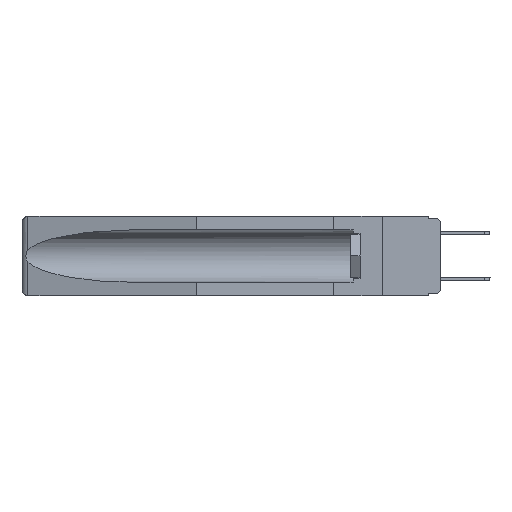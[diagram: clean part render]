
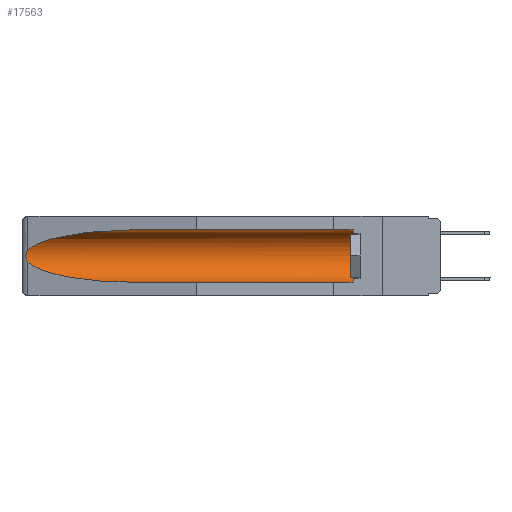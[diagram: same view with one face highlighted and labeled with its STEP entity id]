
A CAD part, left-side view. The second image highlights one B-rep face of the part: STEP entity #17563.
In plain terms, the highlighted cylindrical face has radius 2.857 mm (diameter 5.715 mm), a partial arc.
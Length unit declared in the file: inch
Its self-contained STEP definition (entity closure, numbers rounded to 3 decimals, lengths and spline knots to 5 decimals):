
#345 = EDGE_CURVE ( 'NONE', #7785, #2218, #491, .T. ) ;
#491 =( BOUNDED_CURVE ( )  B_SPLINE_CURVE ( 3, ( #11418, #5272, #18903, #6684 ),
 .UNSPECIFIED., .F., .F. ) 
 B_SPLINE_CURVE_WITH_KNOTS ( ( 4, 4 ),
 ( 4.71239, 6.08839 ),
 .UNSPECIFIED. ) 
 CURVE ( )  GEOMETRIC_REPRESENTATION_ITEM ( )  RATIONAL_B_SPLINE_CURVE ( ( 1., 0.848, 0.848, 1. ) ) 
 REPRESENTATION_ITEM ( '' )  );
#539 = VECTOR ( 'NONE', #11460, 39.37008 ) ;
#713 = CARTESIAN_POINT ( 'NONE',  ( 0.155, -0.30754, -0.284 ) ) ;
#914 = EDGE_CURVE ( 'NONE', #5706, #6888, #1762, .T. ) ;
#940 = EDGE_CURVE ( 'NONE', #5706, #18076, #4893, .T. ) ;
#1762 = CIRCLE ( 'NONE', #2963, 0.1125 ) ;
#1925 = LINE ( 'NONE', #9949, #17726 ) ;
#2218 = VERTEX_POINT ( 'NONE', #7419 ) ;
#2226 = DIRECTION ( 'NONE',  ( 0., 0., 1. ) ) ;
#2325 = DIRECTION ( 'NONE',  ( 0., 0., 1. ) ) ;
#2847 = CARTESIAN_POINT ( 'NONE',  ( 0.26537, 1.52718, -0.19328 ) ) ;
#2963 = AXIS2_PLACEMENT_3D ( 'NONE', #9897, #11526, #2226 ) ;
#3067 = CARTESIAN_POINT ( 'NONE',  ( 0.26537, 1.52718, -0.19328 ) ) ;
#3264 = EDGE_CURVE ( 'NONE', #6962, #18076, #4589, .T. ) ;
#3426 = AXIS2_PLACEMENT_3D ( 'NONE', #16192, #5473, #2325 ) ;
#4138 = EDGE_CURVE ( 'NONE', #2218, #6962, #8749, .T. ) ;
#4213 = CARTESIAN_POINT ( 'NONE',  ( 0.155, 0.126, -0.059 ) ) ;
#4589 =( BOUNDED_CURVE ( )  B_SPLINE_CURVE ( 3, ( #16500, #5777, #8777, #11725 ),
 .UNSPECIFIED., .F., .F. ) 
 B_SPLINE_CURVE_WITH_KNOTS ( ( 4, 4 ),
 ( 0.1948, 1.5708 ),
 .UNSPECIFIED. ) 
 CURVE ( )  GEOMETRIC_REPRESENTATION_ITEM ( )  RATIONAL_B_SPLINE_CURVE ( ( 1., 0.848, 0.848, 1. ) ) 
 REPRESENTATION_ITEM ( '' )  );
#4893 = LINE ( 'NONE', #713, #539 ) ;
#4951 = ORIENTED_EDGE ( 'NONE', *, *, #345, .T. ) ;
#4993 = ORIENTED_EDGE ( 'NONE', *, *, #940, .F. ) ;
#5272 = CARTESIAN_POINT ( 'NONE',  ( 0.21114, 1.30732, -0.059 ) ) ;
#5427 = DIRECTION ( 'NONE',  ( 0., 1., 0. ) ) ;
#5473 = DIRECTION ( 'NONE',  ( 0., 1., 0. ) ) ;
#5706 = VERTEX_POINT ( 'NONE', #11682 ) ;
#5707 = ORIENTED_EDGE ( 'NONE', *, *, #914, .T. ) ;
#5777 = CARTESIAN_POINT ( 'NONE',  ( 0.25451, 1.48313, -0.24835 ) ) ;
#5871 = CARTESIAN_POINT ( 'NONE',  ( 0.155, 1.07973, -0.059 ) ) ;
#6684 = CARTESIAN_POINT ( 'NONE',  ( 0.26537, 1.52718, -0.14972 ) ) ;
#6879 = ORIENTED_EDGE ( 'NONE', *, *, #16979, .T. ) ;
#6888 = VERTEX_POINT ( 'NONE', #4213 ) ;
#6962 = VERTEX_POINT ( 'NONE', #3067 ) ;
#7298 = ORIENTED_EDGE ( 'NONE', *, *, #4138, .T. ) ;
#7402 = CARTESIAN_POINT ( 'NONE',  ( 0.2675, 1.53308, -0.16763 ) ) ;
#7419 = CARTESIAN_POINT ( 'NONE',  ( 0.26537, 1.52718, -0.14972 ) ) ;
#7785 = VERTEX_POINT ( 'NONE', #5871 ) ;
#8699 = EDGE_LOOP ( 'NONE', ( #4951, #7298, #11663, #4993, #5707, #6879 ) ) ;
#8749 = B_SPLINE_CURVE_WITH_KNOTS ( 'NONE', 3,
 ( #19561, #15119, #11794, #8850, #7402, #16447, #10255, #13394, #14923, #2847 ),
 .UNSPECIFIED., .F., .F.,
 ( 4, 2, 2, 2, 4 ),
 ( 0., 0.00029, 0.00058, 0.00087, 0.00117 ),
 .UNSPECIFIED. ) ;
#8777 = CARTESIAN_POINT ( 'NONE',  ( 0.21114, 1.30732, -0.284 ) ) ;
#8850 = CARTESIAN_POINT ( 'NONE',  ( 0.2673, 1.5327, -0.16383 ) ) ;
#9897 = CARTESIAN_POINT ( 'NONE',  ( 0.155, 0.126, -0.1715 ) ) ;
#9949 = CARTESIAN_POINT ( 'NONE',  ( 0.155, -0.30754, -0.059 ) ) ;
#10255 = CARTESIAN_POINT ( 'NONE',  ( 0.2673, 1.53269, -0.17917 ) ) ;
#11418 = CARTESIAN_POINT ( 'NONE',  ( 0.155, 1.07973, -0.059 ) ) ;
#11460 = DIRECTION ( 'NONE',  ( 0., 1., 0. ) ) ;
#11526 = DIRECTION ( 'NONE',  ( 0., -1., 0. ) ) ;
#11663 = ORIENTED_EDGE ( 'NONE', *, *, #3264, .T. ) ;
#11682 = CARTESIAN_POINT ( 'NONE',  ( 0.155, 0.126, -0.284 ) ) ;
#11725 = CARTESIAN_POINT ( 'NONE',  ( 0.155, 1.07973, -0.284 ) ) ;
#11794 = CARTESIAN_POINT ( 'NONE',  ( 0.26654, 1.53092, -0.15636 ) ) ;
#12454 = CARTESIAN_POINT ( 'NONE',  ( 0.155, 1.07973, -0.284 ) ) ;
#13394 = CARTESIAN_POINT ( 'NONE',  ( 0.26655, 1.53094, -0.18657 ) ) ;
#14923 = CARTESIAN_POINT ( 'NONE',  ( 0.26597, 1.5296, -0.19026 ) ) ;
#15119 = CARTESIAN_POINT ( 'NONE',  ( 0.26597, 1.52961, -0.15275 ) ) ;
#15515 = FACE_OUTER_BOUND ( 'NONE', #8699, .T. ) ;
#16192 = CARTESIAN_POINT ( 'NONE',  ( 0.155, -0.30754, -0.1715 ) ) ;
#16447 = CARTESIAN_POINT ( 'NONE',  ( 0.2675, 1.53308, -0.17534 ) ) ;
#16500 = CARTESIAN_POINT ( 'NONE',  ( 0.26537, 1.52718, -0.19328 ) ) ;
#16979 = EDGE_CURVE ( 'NONE', #6888, #7785, #1925, .T. ) ;
#17563 = ADVANCED_FACE ( 'NONE', ( #15515 ), #18414, .F. ) ;
#17726 = VECTOR ( 'NONE', #5427, 39.37008 ) ;
#18076 = VERTEX_POINT ( 'NONE', #12454 ) ;
#18414 = CYLINDRICAL_SURFACE ( 'NONE', #3426, 0.1125 ) ;
#18903 = CARTESIAN_POINT ( 'NONE',  ( 0.25451, 1.48313, -0.09465 ) ) ;
#19561 = CARTESIAN_POINT ( 'NONE',  ( 0.26537, 1.52718, -0.14972 ) ) ;
